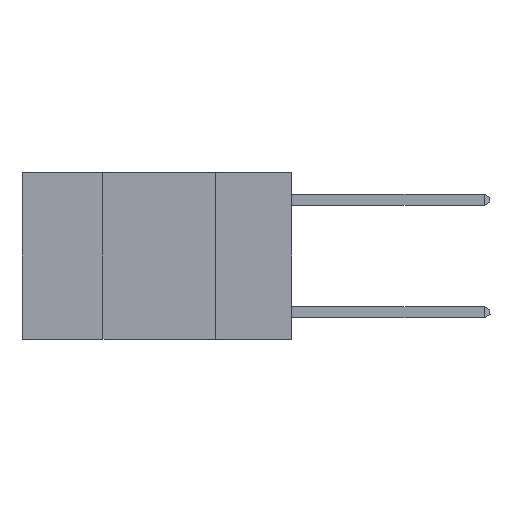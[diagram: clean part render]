
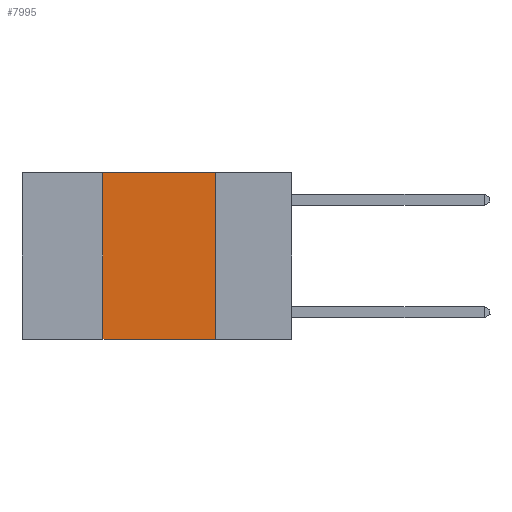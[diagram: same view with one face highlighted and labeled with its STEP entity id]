
A CAD part, left-side view. The second image highlights one B-rep face of the part: STEP entity #7995.
In plain terms, the highlighted planar face has unit normal (-1, 0, 0).
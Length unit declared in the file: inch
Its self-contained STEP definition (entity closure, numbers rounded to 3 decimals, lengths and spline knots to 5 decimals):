
#50 = DIRECTION ( 'NONE',  ( 0., 0., -1. ) ) ;
#109 = CARTESIAN_POINT ( 'NONE',  ( 0., 0.42, -0.37 ) ) ;
#765 = ORIENTED_EDGE ( 'NONE', *, *, #15493, .T. ) ;
#936 = ORIENTED_EDGE ( 'NONE', *, *, #12841, .F. ) ;
#940 = ORIENTED_EDGE ( 'NONE', *, *, #5245, .F. ) ;
#1399 = EDGE_LOOP ( 'NONE', ( #20443, #940, #936, #765 ) ) ;
#1747 = LINE ( 'NONE', #22766, #21753 ) ;
#1930 = FACE_OUTER_BOUND ( 'NONE', #1399, .T. ) ;
#2910 = DIRECTION ( 'NONE',  ( 0., 0., 1. ) ) ;
#2951 = VERTEX_POINT ( 'NONE', #23331 ) ;
#3024 = DIRECTION ( 'NONE',  ( 1., 0., 0. ) ) ;
#3291 = VECTOR ( 'NONE', #50, 39.37008 ) ;
#5245 = EDGE_CURVE ( 'NONE', #7208, #24945, #8101, .T. ) ;
#7208 = VERTEX_POINT ( 'NONE', #19046 ) ;
#7630 = CARTESIAN_POINT ( 'NONE',  ( 0., 0.6, 0. ) ) ;
#7995 = ADVANCED_FACE ( 'NONE', ( #1930 ), #15094, .F. ) ;
#8101 = LINE ( 'NONE', #7630, #12835 ) ;
#12835 = VECTOR ( 'NONE', #15678, 39.37008 ) ;
#12841 = EDGE_CURVE ( 'NONE', #19388, #7208, #1747, .T. ) ;
#13370 = VECTOR ( 'NONE', #15981, 39.37008 ) ;
#14046 = LINE ( 'NONE', #14259, #3291 ) ;
#14259 = CARTESIAN_POINT ( 'NONE',  ( 0., 0.17, 0. ) ) ;
#15094 = PLANE ( 'NONE',  #18185 ) ;
#15493 = EDGE_CURVE ( 'NONE', #19388, #2951, #23733, .T. ) ;
#15678 = DIRECTION ( 'NONE',  ( 0., -1., 0. ) ) ;
#15981 = DIRECTION ( 'NONE',  ( 0., -1., 0. ) ) ;
#17111 = DIRECTION ( 'NONE',  ( 0., 0., -1. ) ) ;
#17836 = CARTESIAN_POINT ( 'NONE',  ( 0., 0.17, 0. ) ) ;
#18185 = AXIS2_PLACEMENT_3D ( 'NONE', #20912, #3024, #17111 ) ;
#19046 = CARTESIAN_POINT ( 'NONE',  ( 0., 0.42, 0. ) ) ;
#19388 = VERTEX_POINT ( 'NONE', #109 ) ;
#20443 = ORIENTED_EDGE ( 'NONE', *, *, #22053, .F. ) ;
#20912 = CARTESIAN_POINT ( 'NONE',  ( 0., 0.6, 0. ) ) ;
#21753 = VECTOR ( 'NONE', #2910, 39.37008 ) ;
#22053 = EDGE_CURVE ( 'NONE', #24945, #2951, #14046, .T. ) ;
#22766 = CARTESIAN_POINT ( 'NONE',  ( 0., 0.42, 0. ) ) ;
#23331 = CARTESIAN_POINT ( 'NONE',  ( 0., 0.17, -0.37 ) ) ;
#23733 = LINE ( 'NONE', #25551, #13370 ) ;
#24945 = VERTEX_POINT ( 'NONE', #17836 ) ;
#25551 = CARTESIAN_POINT ( 'NONE',  ( 0., 0.6, -0.37 ) ) ;
